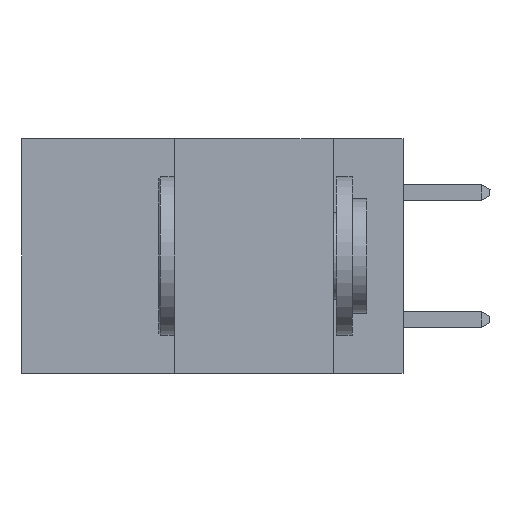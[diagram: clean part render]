
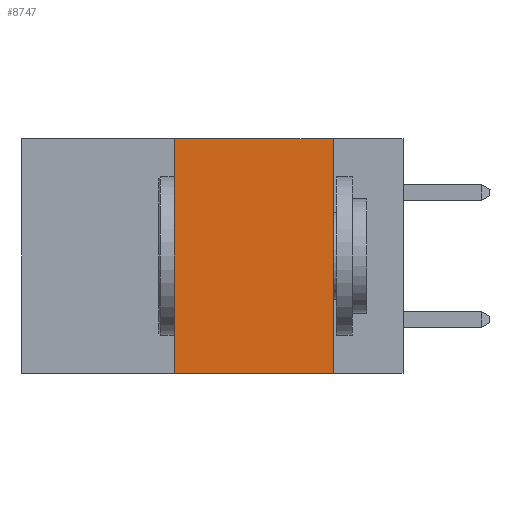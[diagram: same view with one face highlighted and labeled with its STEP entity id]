
A CAD part, left-side view. The second image highlights one B-rep face of the part: STEP entity #8747.
In plain terms, the highlighted planar face has unit normal (-1, 0, 0).
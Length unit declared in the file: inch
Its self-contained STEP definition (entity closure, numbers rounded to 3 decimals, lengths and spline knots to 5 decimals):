
#85 = VECTOR ( 'NONE', #9707, 39.37008 ) ;
#145 = CARTESIAN_POINT ( 'NONE',  ( 0., 0.36, 0. ) ) ;
#531 = PLANE ( 'NONE',  #6693 ) ;
#1876 = CARTESIAN_POINT ( 'NONE',  ( 0., 0.6, 0. ) ) ;
#2480 = VERTEX_POINT ( 'NONE', #7595 ) ;
#2724 = VERTEX_POINT ( 'NONE', #4459 ) ;
#3208 = ORIENTED_EDGE ( 'NONE', *, *, #3945, .F. ) ;
#3491 = VERTEX_POINT ( 'NONE', #4675 ) ;
#3945 = EDGE_CURVE ( 'NONE', #2480, #3491, #11225, .T. ) ;
#4303 = EDGE_CURVE ( 'NONE', #2480, #8900, #9563, .T. ) ;
#4396 = CARTESIAN_POINT ( 'NONE',  ( 0., 0.11, -0.37 ) ) ;
#4459 = CARTESIAN_POINT ( 'NONE',  ( 0., 0.11, 0. ) ) ;
#4611 = DIRECTION ( 'NONE',  ( 0., 0., 1. ) ) ;
#4675 = CARTESIAN_POINT ( 'NONE',  ( 0., 0.36, 0. ) ) ;
#4729 = FACE_OUTER_BOUND ( 'NONE', #4759, .T. ) ;
#4754 = LINE ( 'NONE', #9636, #11623 ) ;
#4759 = EDGE_LOOP ( 'NONE', ( #11288, #10599, #3208, #8016 ) ) ;
#4930 = EDGE_CURVE ( 'NONE', #2724, #8900, #4754, .T. ) ;
#6693 = AXIS2_PLACEMENT_3D ( 'NONE', #8557, #11275, #11315 ) ;
#6863 = DIRECTION ( 'NONE',  ( 0., 0., -1. ) ) ;
#7595 = CARTESIAN_POINT ( 'NONE',  ( 0., 0.36, -0.37 ) ) ;
#8016 = ORIENTED_EDGE ( 'NONE', *, *, #4303, .T. ) ;
#8063 = DIRECTION ( 'NONE',  ( 0., -1., 0. ) ) ;
#8181 = VECTOR ( 'NONE', #4611, 39.37008 ) ;
#8242 = LINE ( 'NONE', #1876, #9356 ) ;
#8557 = CARTESIAN_POINT ( 'NONE',  ( 0., 0.6, 0. ) ) ;
#8747 = ADVANCED_FACE ( 'NONE', ( #4729 ), #531, .F. ) ;
#8900 = VERTEX_POINT ( 'NONE', #4396 ) ;
#9323 = EDGE_CURVE ( 'NONE', #3491, #2724, #8242, .T. ) ;
#9356 = VECTOR ( 'NONE', #8063, 39.37008 ) ;
#9563 = LINE ( 'NONE', #9748, #85 ) ;
#9636 = CARTESIAN_POINT ( 'NONE',  ( 0., 0.11, 0. ) ) ;
#9707 = DIRECTION ( 'NONE',  ( 0., -1., 0. ) ) ;
#9748 = CARTESIAN_POINT ( 'NONE',  ( 0., 0.6, -0.37 ) ) ;
#10599 = ORIENTED_EDGE ( 'NONE', *, *, #9323, .F. ) ;
#11225 = LINE ( 'NONE', #145, #8181 ) ;
#11275 = DIRECTION ( 'NONE',  ( 1., 0., 0. ) ) ;
#11288 = ORIENTED_EDGE ( 'NONE', *, *, #4930, .F. ) ;
#11315 = DIRECTION ( 'NONE',  ( 0., 0., -1. ) ) ;
#11623 = VECTOR ( 'NONE', #6863, 39.37008 ) ;
